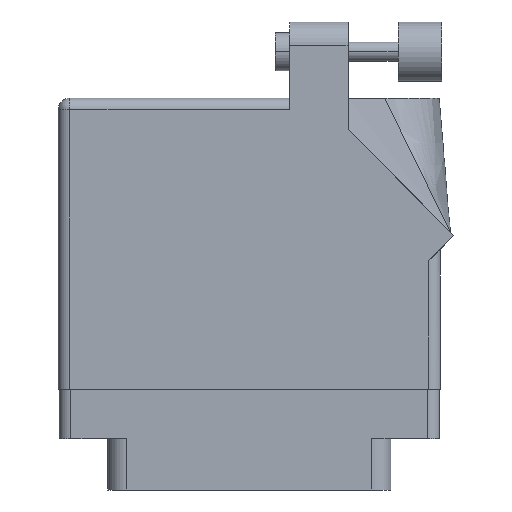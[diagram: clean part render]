
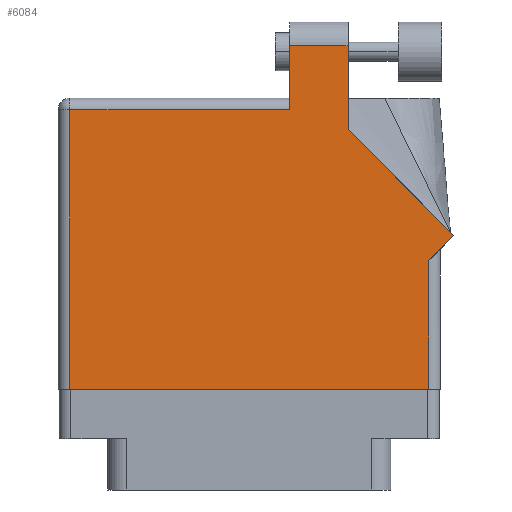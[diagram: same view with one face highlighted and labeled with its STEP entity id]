
A CAD part, front view. The second image highlights one B-rep face of the part: STEP entity #6084.
In plain terms, the highlighted face is planar.
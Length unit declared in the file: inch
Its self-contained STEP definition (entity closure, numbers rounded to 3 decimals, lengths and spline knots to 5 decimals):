
#803 = DIRECTION ( 'NONE',  ( 0., -1., 0. ) ) ;
#1015 = EDGE_CURVE ( 'NONE', #14903, #19391, #27326, .T. ) ;
#1800 = DIRECTION ( 'NONE',  ( -1., 0., 0. ) ) ;
#2190 = ORIENTED_EDGE ( 'NONE', *, *, #1015, .T. ) ;
#3353 = AXIS2_PLACEMENT_3D ( 'NONE', #28038, #28565, #1800 ) ;
#3691 = EDGE_CURVE ( 'NONE', #16394, #37708, #25250, .T. ) ;
#4247 = ORIENTED_EDGE ( 'NONE', *, *, #22725, .T. ) ;
#4298 = DIRECTION ( 'NONE',  ( 0., 1., 0. ) ) ;
#5127 = DIRECTION ( 'NONE',  ( 0., 1., 0. ) ) ;
#5162 = LINE ( 'NONE', #24954, #30519 ) ;
#5212 = CARTESIAN_POINT ( 'NONE',  ( 1.948, 0.675, 0. ) ) ;
#6009 = DIRECTION ( 'NONE',  ( -1., 0., 0. ) ) ;
#6084 = ADVANCED_FACE ( 'NONE', ( #20317 ), #25042, .F. ) ;
#7507 = CARTESIAN_POINT ( 'NONE',  ( 1.524, 1.805, 0. ) ) ;
#8016 = EDGE_CURVE ( 'NONE', #11026, #21528, #33790, .T. ) ;
#8101 = ORIENTED_EDGE ( 'NONE', *, *, #37324, .T. ) ;
#8191 = VECTOR ( 'NONE', #20864, 39.37008 ) ;
#8376 = VECTOR ( 'NONE', #18751, 39.37008 ) ;
#8860 = CARTESIAN_POINT ( 'NONE',  ( 1.217, 1.468, 0. ) ) ;
#9192 = CARTESIAN_POINT ( 'NONE',  ( 1.948, 0., 0. ) ) ;
#9423 = CARTESIAN_POINT ( 'NONE',  ( 1.217, 1.805, 0. ) ) ;
#9488 = CARTESIAN_POINT ( 'NONE',  ( 1.217, 1.53, 0. ) ) ;
#9515 = CARTESIAN_POINT ( 'NONE',  ( 0., 1.468, 0. ) ) ;
#9858 = CARTESIAN_POINT ( 'NONE',  ( 0.062, 0., 0. ) ) ;
#11026 = VERTEX_POINT ( 'NONE', #8860 ) ;
#11883 = VECTOR ( 'NONE', #6009, 39.37008 ) ;
#13550 = ORIENTED_EDGE ( 'NONE', *, *, #26314, .T. ) ;
#13587 = EDGE_LOOP ( 'NONE', ( #15141, #21036, #28062, #31871, #20547, #4247, #2190, #8101, #13550 ) ) ;
#13594 = LINE ( 'NONE', #9488, #18767 ) ;
#14686 = CARTESIAN_POINT ( 'NONE',  ( 2.08071, 0.80771, 0. ) ) ;
#14903 = VERTEX_POINT ( 'NONE', #9192 ) ;
#15141 = ORIENTED_EDGE ( 'NONE', *, *, #3691, .T. ) ;
#15580 = LINE ( 'NONE', #9858, #33926 ) ;
#16210 = LINE ( 'NONE', #38751, #8191 ) ;
#16394 = VERTEX_POINT ( 'NONE', #22211 ) ;
#18751 = DIRECTION ( 'NONE',  ( -1., 0., 0. ) ) ;
#18767 = VECTOR ( 'NONE', #24881, 39.37008 ) ;
#19391 = VERTEX_POINT ( 'NONE', #5212 ) ;
#19407 = VECTOR ( 'NONE', #5127, 39.37008 ) ;
#19597 = EDGE_CURVE ( 'NONE', #26908, #11026, #13594, .T. ) ;
#19807 = CARTESIAN_POINT ( 'NONE',  ( 1.217, 1.805, 0. ) ) ;
#20317 = FACE_OUTER_BOUND ( 'NONE', #13587, .T. ) ;
#20547 = ORIENTED_EDGE ( 'NONE', *, *, #31124, .T. ) ;
#20864 = DIRECTION ( 'NONE',  ( 1., 0., 0. ) ) ;
#21036 = ORIENTED_EDGE ( 'NONE', *, *, #23239, .T. ) ;
#21528 = VERTEX_POINT ( 'NONE', #23178 ) ;
#21727 = LINE ( 'NONE', #38331, #30595 ) ;
#22090 = VERTEX_POINT ( 'NONE', #37510 ) ;
#22211 = CARTESIAN_POINT ( 'NONE',  ( 1.524, 1.36442, 0. ) ) ;
#22578 = CARTESIAN_POINT ( 'NONE',  ( 1.524, 1.36442, 0. ) ) ;
#22725 = EDGE_CURVE ( 'NONE', #22090, #14903, #16210, .T. ) ;
#22767 = CARTESIAN_POINT ( 'NONE',  ( 1.948, 0.737, 0. ) ) ;
#23178 = CARTESIAN_POINT ( 'NONE',  ( 0.062, 1.468, 0. ) ) ;
#23239 = EDGE_CURVE ( 'NONE', #37708, #26908, #37815, .T. ) ;
#24881 = DIRECTION ( 'NONE',  ( 0., -1., 0. ) ) ;
#24954 = CARTESIAN_POINT ( 'NONE',  ( 2.08071, 0.80771, 0. ) ) ;
#25042 = PLANE ( 'NONE',  #3353 ) ;
#25250 = LINE ( 'NONE', #22578, #38917 ) ;
#26314 = EDGE_CURVE ( 'NONE', #36750, #16394, #5162, .T. ) ;
#26908 = VERTEX_POINT ( 'NONE', #19807 ) ;
#27326 = LINE ( 'NONE', #22767, #19407 ) ;
#28038 = CARTESIAN_POINT ( 'NONE',  ( 0., 1.53, 0. ) ) ;
#28062 = ORIENTED_EDGE ( 'NONE', *, *, #19597, .T. ) ;
#28072 = DIRECTION ( 'NONE',  ( -0.707, 0.707, 0. ) ) ;
#28565 = DIRECTION ( 'NONE',  ( 0., 0., -1. ) ) ;
#30519 = VECTOR ( 'NONE', #28072, 39.37008 ) ;
#30595 = VECTOR ( 'NONE', #38843, 39.37008 ) ;
#31124 = EDGE_CURVE ( 'NONE', #21528, #22090, #15580, .T. ) ;
#31871 = ORIENTED_EDGE ( 'NONE', *, *, #8016, .T. ) ;
#33790 = LINE ( 'NONE', #9515, #8376 ) ;
#33926 = VECTOR ( 'NONE', #803, 39.37008 ) ;
#36750 = VERTEX_POINT ( 'NONE', #14686 ) ;
#37324 = EDGE_CURVE ( 'NONE', #19391, #36750, #21727, .T. ) ;
#37510 = CARTESIAN_POINT ( 'NONE',  ( 0.062, 0., 0. ) ) ;
#37708 = VERTEX_POINT ( 'NONE', #7507 ) ;
#37815 = LINE ( 'NONE', #9423, #11883 ) ;
#38331 = CARTESIAN_POINT ( 'NONE',  ( 2.01, 0.737, 0. ) ) ;
#38751 = CARTESIAN_POINT ( 'NONE',  ( 0., 0., 0. ) ) ;
#38843 = DIRECTION ( 'NONE',  ( 0.707, 0.707, 0. ) ) ;
#38917 = VECTOR ( 'NONE', #4298, 39.37008 ) ;
